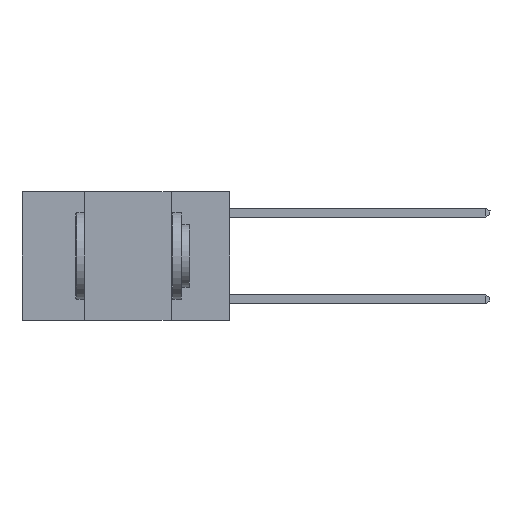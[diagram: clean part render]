
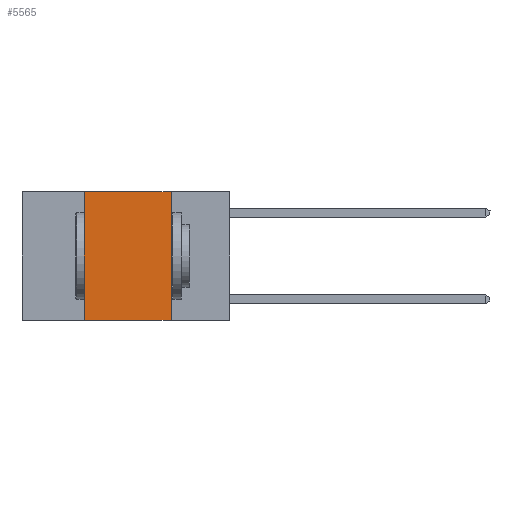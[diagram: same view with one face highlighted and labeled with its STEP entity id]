
A CAD part, left-side view. The second image highlights one B-rep face of the part: STEP entity #5565.
In plain terms, the highlighted planar face has unit normal (-1, 0, 0).
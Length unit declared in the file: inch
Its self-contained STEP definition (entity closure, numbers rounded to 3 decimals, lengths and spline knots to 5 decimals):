
#157 = DIRECTION ( 'NONE',  ( 0., -1., 0. ) ) ;
#220 = CARTESIAN_POINT ( 'NONE',  ( 0., 0.6, -0.37 ) ) ;
#280 = VECTOR ( 'NONE', #7765, 39.37008 ) ;
#540 = LINE ( 'NONE', #929, #280 ) ;
#555 = EDGE_CURVE ( 'NONE', #4038, #4742, #6277, .T. ) ;
#929 = CARTESIAN_POINT ( 'NONE',  ( 0., 0.17, 0. ) ) ;
#1071 = DIRECTION ( 'NONE',  ( 1., 0., 0. ) ) ;
#1189 = EDGE_CURVE ( 'NONE', #4742, #1603, #540, .T. ) ;
#1603 = VERTEX_POINT ( 'NONE', #6219 ) ;
#1661 = ORIENTED_EDGE ( 'NONE', *, *, #2372, .F. ) ;
#1964 = CARTESIAN_POINT ( 'NONE',  ( 0., 0.6, 0. ) ) ;
#2185 = FACE_OUTER_BOUND ( 'NONE', #7172, .T. ) ;
#2247 = VERTEX_POINT ( 'NONE', #4165 ) ;
#2372 = EDGE_CURVE ( 'NONE', #2247, #4038, #9055, .T. ) ;
#2913 = ORIENTED_EDGE ( 'NONE', *, *, #555, .F. ) ;
#2984 = VECTOR ( 'NONE', #7340, 39.37008 ) ;
#4038 = VERTEX_POINT ( 'NONE', #4330 ) ;
#4106 = VECTOR ( 'NONE', #7025, 39.37008 ) ;
#4165 = CARTESIAN_POINT ( 'NONE',  ( 0., 0.42, -0.37 ) ) ;
#4214 = EDGE_CURVE ( 'NONE', #2247, #1603, #4362, .T. ) ;
#4330 = CARTESIAN_POINT ( 'NONE',  ( 0., 0.42, 0. ) ) ;
#4362 = LINE ( 'NONE', #220, #5852 ) ;
#4526 = ORIENTED_EDGE ( 'NONE', *, *, #1189, .F. ) ;
#4742 = VERTEX_POINT ( 'NONE', #9321 ) ;
#5565 = ADVANCED_FACE ( 'NONE', ( #2185 ), #8481, .F. ) ;
#5591 = CARTESIAN_POINT ( 'NONE',  ( 0., 0.6, 0. ) ) ;
#5852 = VECTOR ( 'NONE', #157, 39.37008 ) ;
#6219 = CARTESIAN_POINT ( 'NONE',  ( 0., 0.17, -0.37 ) ) ;
#6277 = LINE ( 'NONE', #1964, #4106 ) ;
#6308 = DIRECTION ( 'NONE',  ( 0., 0., -1. ) ) ;
#7025 = DIRECTION ( 'NONE',  ( 0., -1., 0. ) ) ;
#7172 = EDGE_LOOP ( 'NONE', ( #4526, #2913, #1661, #9403 ) ) ;
#7340 = DIRECTION ( 'NONE',  ( 0., 0., 1. ) ) ;
#7671 = CARTESIAN_POINT ( 'NONE',  ( 0., 0.42, 0. ) ) ;
#7765 = DIRECTION ( 'NONE',  ( 0., 0., -1. ) ) ;
#8131 = AXIS2_PLACEMENT_3D ( 'NONE', #5591, #1071, #6308 ) ;
#8481 = PLANE ( 'NONE',  #8131 ) ;
#9055 = LINE ( 'NONE', #7671, #2984 ) ;
#9321 = CARTESIAN_POINT ( 'NONE',  ( 0., 0.17, 0. ) ) ;
#9403 = ORIENTED_EDGE ( 'NONE', *, *, #4214, .T. ) ;
